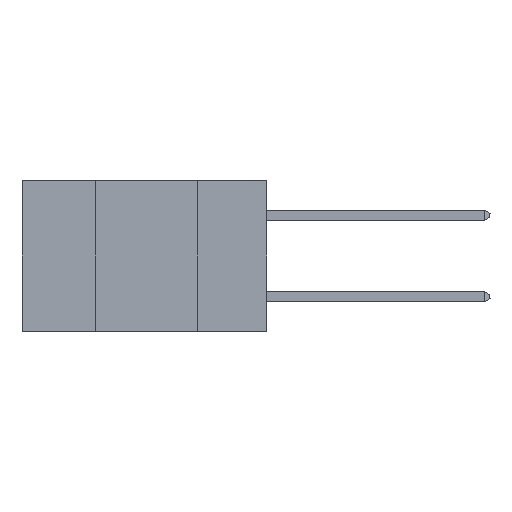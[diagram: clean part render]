
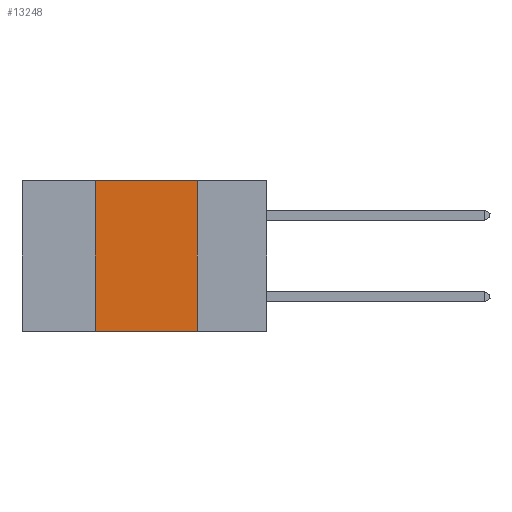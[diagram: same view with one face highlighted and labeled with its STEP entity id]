
A CAD part, left-side view. The second image highlights one B-rep face of the part: STEP entity #13248.
In plain terms, the highlighted planar face has unit normal (-1, 0, 0).
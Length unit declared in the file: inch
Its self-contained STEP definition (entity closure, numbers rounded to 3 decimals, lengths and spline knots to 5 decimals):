
#293 = VECTOR ( 'NONE', #15829, 39.37008 ) ;
#1972 = VERTEX_POINT ( 'NONE', #11473 ) ;
#2082 = FACE_OUTER_BOUND ( 'NONE', #18143, .T. ) ;
#3390 = ORIENTED_EDGE ( 'NONE', *, *, #21450, .F. ) ;
#3551 = VECTOR ( 'NONE', #7610, 39.37008 ) ;
#3657 = CARTESIAN_POINT ( 'NONE',  ( 0., 0.42, 0. ) ) ;
#3975 = EDGE_CURVE ( 'NONE', #20456, #5831, #21391, .T. ) ;
#4990 = LINE ( 'NONE', #14484, #18738 ) ;
#5177 = LINE ( 'NONE', #14024, #293 ) ;
#5545 = DIRECTION ( 'NONE',  ( 0., 0., -1. ) ) ;
#5808 = DIRECTION ( 'NONE',  ( 0., 0., -1. ) ) ;
#5810 = CARTESIAN_POINT ( 'NONE',  ( 0., 0.6, -0.37 ) ) ;
#5831 = VERTEX_POINT ( 'NONE', #7447 ) ;
#7447 = CARTESIAN_POINT ( 'NONE',  ( 0., 0.17, -0.37 ) ) ;
#7522 = CARTESIAN_POINT ( 'NONE',  ( 0., 0.17, 0. ) ) ;
#7610 = DIRECTION ( 'NONE',  ( 0., -1., 0. ) ) ;
#8015 = EDGE_CURVE ( 'NONE', #1972, #8570, #4990, .T. ) ;
#8570 = VERTEX_POINT ( 'NONE', #3657 ) ;
#9142 = DIRECTION ( 'NONE',  ( 0., 0., 1. ) ) ;
#10385 = ORIENTED_EDGE ( 'NONE', *, *, #8015, .F. ) ;
#11213 = ORIENTED_EDGE ( 'NONE', *, *, #3975, .F. ) ;
#11473 = CARTESIAN_POINT ( 'NONE',  ( 0., 0.42, -0.37 ) ) ;
#12641 = EDGE_CURVE ( 'NONE', #1972, #5831, #17869, .T. ) ;
#12673 = CARTESIAN_POINT ( 'NONE',  ( 0., 0.6, 0. ) ) ;
#13248 = ADVANCED_FACE ( 'NONE', ( #2082 ), #21587, .F. ) ;
#14024 = CARTESIAN_POINT ( 'NONE',  ( 0., 0.6, 0. ) ) ;
#14484 = CARTESIAN_POINT ( 'NONE',  ( 0., 0.42, 0. ) ) ;
#15829 = DIRECTION ( 'NONE',  ( 0., -1., 0. ) ) ;
#16307 = DIRECTION ( 'NONE',  ( 1., 0., 0. ) ) ;
#17430 = ORIENTED_EDGE ( 'NONE', *, *, #12641, .T. ) ;
#17869 = LINE ( 'NONE', #5810, #3551 ) ;
#18143 = EDGE_LOOP ( 'NONE', ( #11213, #3390, #10385, #17430 ) ) ;
#18607 = CARTESIAN_POINT ( 'NONE',  ( 0., 0.17, 0. ) ) ;
#18738 = VECTOR ( 'NONE', #9142, 39.37008 ) ;
#18757 = AXIS2_PLACEMENT_3D ( 'NONE', #12673, #16307, #5545 ) ;
#20456 = VERTEX_POINT ( 'NONE', #18607 ) ;
#20836 = VECTOR ( 'NONE', #5808, 39.37008 ) ;
#21391 = LINE ( 'NONE', #7522, #20836 ) ;
#21450 = EDGE_CURVE ( 'NONE', #8570, #20456, #5177, .T. ) ;
#21587 = PLANE ( 'NONE',  #18757 ) ;
